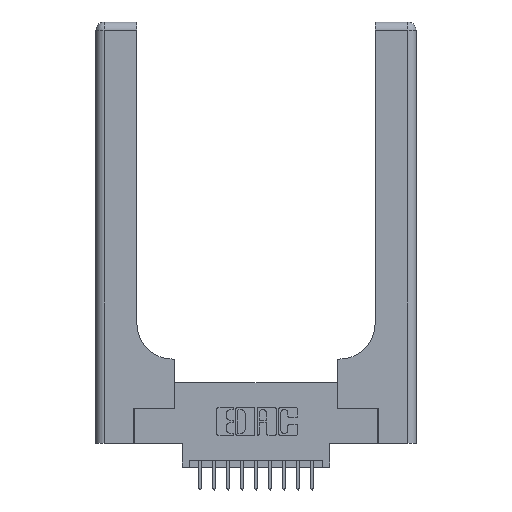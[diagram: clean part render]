
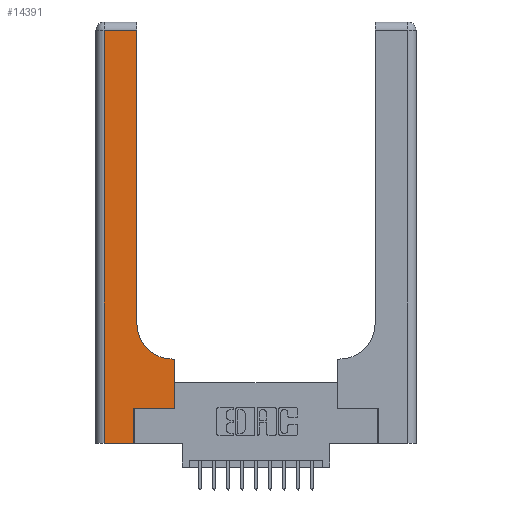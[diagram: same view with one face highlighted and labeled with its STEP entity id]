
A CAD part, top view. The second image highlights one B-rep face of the part: STEP entity #14391.
In plain terms, the highlighted planar face has unit normal (0, 0, 1).
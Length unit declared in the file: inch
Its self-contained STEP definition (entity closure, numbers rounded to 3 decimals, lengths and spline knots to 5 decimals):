
#19 = DIRECTION ( 'NONE',  ( -1., 0., 0. ) ) ;
#257 = VECTOR ( 'NONE', #1230, 39.37008 ) ;
#348 = CARTESIAN_POINT ( 'NONE',  ( 0.06, 3., 0.37 ) ) ;
#479 = LINE ( 'NONE', #348, #10695 ) ;
#694 = CARTESIAN_POINT ( 'NONE',  ( 0.2915, 0.6, 0.37 ) ) ;
#948 = ORIENTED_EDGE ( 'NONE', *, *, #12668, .T. ) ;
#1230 = DIRECTION ( 'NONE',  ( 0., 1., 0. ) ) ;
#2085 = PLANE ( 'NONE',  #12014 ) ;
#2104 = ORIENTED_EDGE ( 'NONE', *, *, #8639, .T. ) ;
#2464 = FACE_OUTER_BOUND ( 'NONE', #10587, .T. ) ;
#2522 = VERTEX_POINT ( 'NONE', #13089 ) ;
#3143 = DIRECTION ( 'NONE',  ( 1., 0., 0. ) ) ;
#3314 = CARTESIAN_POINT ( 'NONE',  ( 0.2915, 0.85, 0.37 ) ) ;
#3641 = DIRECTION ( 'NONE',  ( 0., 0., -1. ) ) ;
#3845 = CARTESIAN_POINT ( 'NONE',  ( 0.269, 0., 0.37 ) ) ;
#3871 = LINE ( 'NONE', #9302, #10361 ) ;
#4030 = LINE ( 'NONE', #8006, #257 ) ;
#4320 = VECTOR ( 'NONE', #19, 39.37008 ) ;
#4324 = ORIENTED_EDGE ( 'NONE', *, *, #10783, .T. ) ;
#4607 = CARTESIAN_POINT ( 'NONE',  ( 0.06, 2.94, 0.37 ) ) ;
#4832 = VERTEX_POINT ( 'NONE', #15441 ) ;
#4853 = DIRECTION ( 'NONE',  ( 0., 0., -1. ) ) ;
#5106 = CIRCLE ( 'NONE', #9066, 0.25 ) ;
#5350 = DIRECTION ( 'NONE',  ( 1., 0., 0. ) ) ;
#5420 = EDGE_CURVE ( 'NONE', #13684, #2522, #12360, .T. ) ;
#5791 = ORIENTED_EDGE ( 'NONE', *, *, #8243, .T. ) ;
#5914 = VERTEX_POINT ( 'NONE', #10178 ) ;
#5938 = VECTOR ( 'NONE', #3143, 39.37008 ) ;
#6544 = LINE ( 'NONE', #3845, #9555 ) ;
#6918 = CARTESIAN_POINT ( 'NONE',  ( 0., 2.94, 0.37 ) ) ;
#7390 = VERTEX_POINT ( 'NONE', #4607 ) ;
#7445 = CARTESIAN_POINT ( 'NONE',  ( 0., 3., 0.37 ) ) ;
#7740 = VERTEX_POINT ( 'NONE', #9255 ) ;
#8006 = CARTESIAN_POINT ( 'NONE',  ( 0.5585, 0.25, 0.37 ) ) ;
#8096 = VERTEX_POINT ( 'NONE', #3314 ) ;
#8177 = EDGE_CURVE ( 'NONE', #4832, #10094, #9374, .T. ) ;
#8243 = EDGE_CURVE ( 'NONE', #10094, #8096, #5106, .T. ) ;
#8435 = CARTESIAN_POINT ( 'NONE',  ( 0.269, 0.25, 0.37 ) ) ;
#8639 = EDGE_CURVE ( 'NONE', #5914, #7740, #9361, .T. ) ;
#8977 = VECTOR ( 'NONE', #12517, 39.37008 ) ;
#9066 = AXIS2_PLACEMENT_3D ( 'NONE', #11390, #3641, #12662 ) ;
#9122 = DIRECTION ( 'NONE',  ( 0., 1., 0. ) ) ;
#9255 = CARTESIAN_POINT ( 'NONE',  ( 0.5585, 0.25, 0.37 ) ) ;
#9302 = CARTESIAN_POINT ( 'NONE',  ( 0.2915, 3., 0.37 ) ) ;
#9361 = LINE ( 'NONE', #8435, #5938 ) ;
#9374 = LINE ( 'NONE', #694, #8977 ) ;
#9442 = VECTOR ( 'NONE', #5350, 39.37008 ) ;
#9555 = VECTOR ( 'NONE', #9122, 39.37008 ) ;
#9687 = CARTESIAN_POINT ( 'NONE',  ( 0.06, 0., 0.37 ) ) ;
#9694 = DIRECTION ( 'NONE',  ( 0., -1., 0. ) ) ;
#10094 = VERTEX_POINT ( 'NONE', #11607 ) ;
#10178 = CARTESIAN_POINT ( 'NONE',  ( 0.269, 0.25, 0.37 ) ) ;
#10237 = EDGE_CURVE ( 'NONE', #15662, #7390, #10777, .T. ) ;
#10304 = ORIENTED_EDGE ( 'NONE', *, *, #11832, .T. ) ;
#10361 = VECTOR ( 'NONE', #16785, 39.37008 ) ;
#10587 = EDGE_LOOP ( 'NONE', ( #4324, #14579, #948, #13616, #10304, #2104, #14766, #16539, #5791 ) ) ;
#10695 = VECTOR ( 'NONE', #9694, 39.37008 ) ;
#10777 = LINE ( 'NONE', #6918, #4320 ) ;
#10783 = EDGE_CURVE ( 'NONE', #8096, #15662, #3871, .T. ) ;
#11390 = CARTESIAN_POINT ( 'NONE',  ( 0.5415, 0.85, 0.37 ) ) ;
#11607 = CARTESIAN_POINT ( 'NONE',  ( 0.5415, 0.6, 0.37 ) ) ;
#11832 = EDGE_CURVE ( 'NONE', #2522, #5914, #6544, .T. ) ;
#12014 = AXIS2_PLACEMENT_3D ( 'NONE', #7445, #4853, #13783 ) ;
#12360 = LINE ( 'NONE', #14237, #9442 ) ;
#12441 = EDGE_CURVE ( 'NONE', #7740, #4832, #4030, .T. ) ;
#12517 = DIRECTION ( 'NONE',  ( -1., 0., 0. ) ) ;
#12662 = DIRECTION ( 'NONE',  ( 1., 0., 0. ) ) ;
#12668 = EDGE_CURVE ( 'NONE', #7390, #13684, #479, .T. ) ;
#13089 = CARTESIAN_POINT ( 'NONE',  ( 0.269, 0., 0.37 ) ) ;
#13616 = ORIENTED_EDGE ( 'NONE', *, *, #5420, .T. ) ;
#13684 = VERTEX_POINT ( 'NONE', #9687 ) ;
#13783 = DIRECTION ( 'NONE',  ( -1., 0., 0. ) ) ;
#14237 = CARTESIAN_POINT ( 'NONE',  ( 0., 0., 0.37 ) ) ;
#14391 = ADVANCED_FACE ( 'NONE', ( #2464 ), #2085, .F. ) ;
#14579 = ORIENTED_EDGE ( 'NONE', *, *, #10237, .T. ) ;
#14710 = CARTESIAN_POINT ( 'NONE',  ( 0.2915, 2.94, 0.37 ) ) ;
#14766 = ORIENTED_EDGE ( 'NONE', *, *, #12441, .T. ) ;
#15441 = CARTESIAN_POINT ( 'NONE',  ( 0.5585, 0.6, 0.37 ) ) ;
#15662 = VERTEX_POINT ( 'NONE', #14710 ) ;
#16539 = ORIENTED_EDGE ( 'NONE', *, *, #8177, .T. ) ;
#16785 = DIRECTION ( 'NONE',  ( 0., 1., 0. ) ) ;
